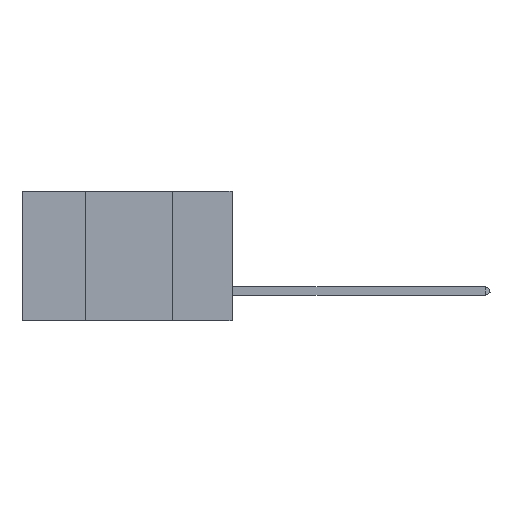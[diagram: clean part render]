
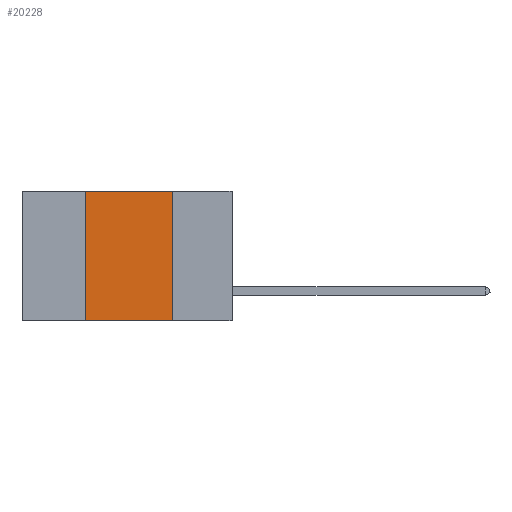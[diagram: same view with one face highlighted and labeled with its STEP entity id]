
A CAD part, left-side view. The second image highlights one B-rep face of the part: STEP entity #20228.
In plain terms, the highlighted planar face has unit normal (-1, 0, 0).
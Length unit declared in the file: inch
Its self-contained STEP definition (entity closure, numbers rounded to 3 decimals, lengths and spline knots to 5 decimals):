
#68 = LINE ( 'NONE', #28069, #5548 ) ;
#1435 = EDGE_CURVE ( 'NONE', #10396, #23389, #23488, .T. ) ;
#1541 = ORIENTED_EDGE ( 'NONE', *, *, #20865, .F. ) ;
#1825 = DIRECTION ( 'NONE',  ( 0., -1., 0. ) ) ;
#3459 = EDGE_LOOP ( 'NONE', ( #25106, #1541, #12442, #18449 ) ) ;
#3952 = LINE ( 'NONE', #16269, #23509 ) ;
#5548 = VECTOR ( 'NONE', #23717, 39.37008 ) ;
#5979 = LINE ( 'NONE', #10498, #13375 ) ;
#8152 = FACE_OUTER_BOUND ( 'NONE', #3459, .T. ) ;
#8989 = CARTESIAN_POINT ( 'NONE',  ( 0., 0.6, -0.37 ) ) ;
#10396 = VERTEX_POINT ( 'NONE', #27044 ) ;
#10498 = CARTESIAN_POINT ( 'NONE',  ( 0., 0.42, 0. ) ) ;
#10804 = EDGE_CURVE ( 'NONE', #12988, #23389, #3952, .T. ) ;
#11663 = VECTOR ( 'NONE', #1825, 39.37008 ) ;
#11722 = CARTESIAN_POINT ( 'NONE',  ( 0., 0.6, 0. ) ) ;
#12442 = ORIENTED_EDGE ( 'NONE', *, *, #13039, .F. ) ;
#12988 = VERTEX_POINT ( 'NONE', #17623 ) ;
#13039 = EDGE_CURVE ( 'NONE', #10396, #26298, #5979, .T. ) ;
#13375 = VECTOR ( 'NONE', #15459, 39.37008 ) ;
#13904 = DIRECTION ( 'NONE',  ( 1., 0., 0. ) ) ;
#13943 = AXIS2_PLACEMENT_3D ( 'NONE', #11722, #13904, #16291 ) ;
#15459 = DIRECTION ( 'NONE',  ( 0., 0., 1. ) ) ;
#16269 = CARTESIAN_POINT ( 'NONE',  ( 0., 0.17, 0. ) ) ;
#16291 = DIRECTION ( 'NONE',  ( 0., 0., -1. ) ) ;
#17623 = CARTESIAN_POINT ( 'NONE',  ( 0., 0.17, 0. ) ) ;
#18208 = DIRECTION ( 'NONE',  ( 0., 0., -1. ) ) ;
#18449 = ORIENTED_EDGE ( 'NONE', *, *, #1435, .T. ) ;
#18618 = CARTESIAN_POINT ( 'NONE',  ( 0., 0.17, -0.37 ) ) ;
#20228 = ADVANCED_FACE ( 'NONE', ( #8152 ), #28134, .F. ) ;
#20865 = EDGE_CURVE ( 'NONE', #26298, #12988, #68, .T. ) ;
#23389 = VERTEX_POINT ( 'NONE', #18618 ) ;
#23488 = LINE ( 'NONE', #8989, #11663 ) ;
#23509 = VECTOR ( 'NONE', #18208, 39.37008 ) ;
#23717 = DIRECTION ( 'NONE',  ( 0., -1., 0. ) ) ;
#25106 = ORIENTED_EDGE ( 'NONE', *, *, #10804, .F. ) ;
#26298 = VERTEX_POINT ( 'NONE', #27220 ) ;
#27044 = CARTESIAN_POINT ( 'NONE',  ( 0., 0.42, -0.37 ) ) ;
#27220 = CARTESIAN_POINT ( 'NONE',  ( 0., 0.42, 0. ) ) ;
#28069 = CARTESIAN_POINT ( 'NONE',  ( 0., 0.6, 0. ) ) ;
#28134 = PLANE ( 'NONE',  #13943 ) ;
